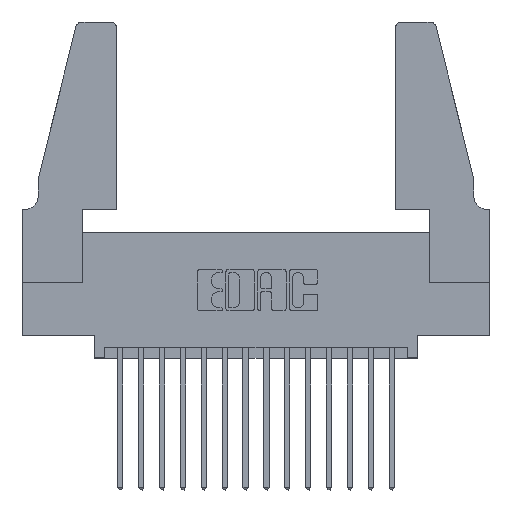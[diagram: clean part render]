
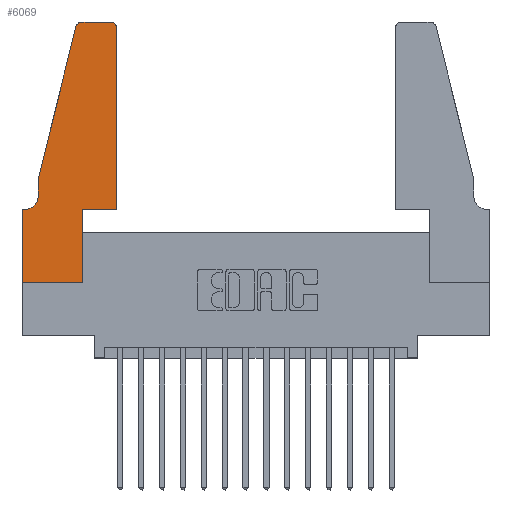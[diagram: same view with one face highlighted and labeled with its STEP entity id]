
A CAD part, top view. The second image highlights one B-rep face of the part: STEP entity #6069.
In plain terms, the highlighted planar face has unit normal (0, 0, 1).
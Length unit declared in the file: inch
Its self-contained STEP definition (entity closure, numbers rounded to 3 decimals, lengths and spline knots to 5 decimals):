
#523 = VERTEX_POINT ( 'NONE', #4623 ) ;
#659 = DIRECTION ( 'NONE',  ( -1., 0., 0. ) ) ;
#923 = DIRECTION ( 'NONE',  ( 1., 0., 0. ) ) ;
#1056 = EDGE_CURVE ( 'NONE', #14252, #4500, #13215, .T. ) ;
#1067 = VERTEX_POINT ( 'NONE', #11701 ) ;
#1222 = ORIENTED_EDGE ( 'NONE', *, *, #1919, .T. ) ;
#1332 = CARTESIAN_POINT ( 'NONE',  ( 0.0755, 0.5, 0.37 ) ) ;
#1691 = VERTEX_POINT ( 'NONE', #14984 ) ;
#1779 = CARTESIAN_POINT ( 'NONE',  ( 0., 0., 0.37 ) ) ;
#1919 = EDGE_CURVE ( 'NONE', #10856, #523, #10089, .T. ) ;
#2397 = VECTOR ( 'NONE', #659, 39.37008 ) ;
#2591 = CARTESIAN_POINT ( 'NONE',  ( 0.4505, 0.35, 0.37 ) ) ;
#2633 = FACE_OUTER_BOUND ( 'NONE', #6565, .T. ) ;
#2664 = ORIENTED_EDGE ( 'NONE', *, *, #2815, .T. ) ;
#2815 = EDGE_CURVE ( 'NONE', #8486, #12716, #12316, .T. ) ;
#3139 = VERTEX_POINT ( 'NONE', #11170 ) ;
#3157 = CARTESIAN_POINT ( 'NONE',  ( 0.284, 1.22, 0.37 ) ) ;
#3527 = VECTOR ( 'NONE', #16235, 39.37008 ) ;
#3567 = CARTESIAN_POINT ( 'NONE',  ( 0.2865, 0.35, 0.37 ) ) ;
#3930 = ORIENTED_EDGE ( 'NONE', *, *, #1056, .T. ) ;
#4178 = CARTESIAN_POINT ( 'NONE',  ( 0.4505, 0.35, 0.37 ) ) ;
#4500 = VERTEX_POINT ( 'NONE', #4964 ) ;
#4520 = DIRECTION ( 'NONE',  ( 1., 0., 0. ) ) ;
#4623 = CARTESIAN_POINT ( 'NONE',  ( 0.2865, 0.35, 0.37 ) ) ;
#4757 = EDGE_CURVE ( 'NONE', #12716, #1067, #7032, .T. ) ;
#4780 = ORIENTED_EDGE ( 'NONE', *, *, #6466, .T. ) ;
#4964 = CARTESIAN_POINT ( 'NONE',  ( 0., 0.35, 0.37 ) ) ;
#5061 = EDGE_CURVE ( 'NONE', #3139, #9304, #5195, .T. ) ;
#5195 = LINE ( 'NONE', #2591, #15659 ) ;
#5306 = EDGE_CURVE ( 'NONE', #13764, #8486, #14652, .T. ) ;
#5380 = CIRCLE ( 'NONE', #12347, 0.07 ) ;
#5598 = DIRECTION ( 'NONE',  ( 0., 0., -1. ) ) ;
#5767 = VECTOR ( 'NONE', #11004, 39.37008 ) ;
#5789 = ORIENTED_EDGE ( 'NONE', *, *, #15074, .T. ) ;
#5987 = DIRECTION ( 'NONE',  ( 0., 0., 1. ) ) ;
#6069 = ADVANCED_FACE ( 'NONE', ( #2633 ), #13903, .T. ) ;
#6105 = DIRECTION ( 'NONE',  ( 0., 0., 1. ) ) ;
#6466 = EDGE_CURVE ( 'NONE', #523, #3139, #11343, .T. ) ;
#6565 = EDGE_LOOP ( 'NONE', ( #5789, #9297, #2664, #6605, #17077, #3930, #7438, #14859, #1222, #4780, #9094, #16058 ) ) ;
#6605 = ORIENTED_EDGE ( 'NONE', *, *, #4757, .T. ) ;
#7032 = LINE ( 'NONE', #14943, #3527 ) ;
#7135 = CARTESIAN_POINT ( 'NONE',  ( 0.284, 1.25, 0.37 ) ) ;
#7438 = ORIENTED_EDGE ( 'NONE', *, *, #14861, .T. ) ;
#7891 = CARTESIAN_POINT ( 'NONE',  ( 0.2865, 0., 0.37 ) ) ;
#8262 = AXIS2_PLACEMENT_3D ( 'NONE', #3157, #12433, #4520 ) ;
#8486 = VERTEX_POINT ( 'NONE', #14629 ) ;
#8613 = CARTESIAN_POINT ( 'NONE',  ( 0.4505, 1.22, 0.37 ) ) ;
#8853 = CARTESIAN_POINT ( 'NONE',  ( 0., 0., 0.37 ) ) ;
#9094 = ORIENTED_EDGE ( 'NONE', *, *, #5061, .T. ) ;
#9297 = ORIENTED_EDGE ( 'NONE', *, *, #5306, .T. ) ;
#9304 = VERTEX_POINT ( 'NONE', #8613 ) ;
#10089 = LINE ( 'NONE', #3567, #10508 ) ;
#10294 = LINE ( 'NONE', #16446, #2397 ) ;
#10508 = VECTOR ( 'NONE', #11502, 39.37008 ) ;
#10517 = VECTOR ( 'NONE', #14729, 39.37008 ) ;
#10621 = EDGE_CURVE ( 'NONE', #9304, #1691, #16713, .T. ) ;
#10639 = CARTESIAN_POINT ( 'NONE',  ( 0.0755, 0.35, 0.37 ) ) ;
#10856 = VERTEX_POINT ( 'NONE', #7891 ) ;
#11004 = DIRECTION ( 'NONE',  ( -1., 0., 0. ) ) ;
#11170 = CARTESIAN_POINT ( 'NONE',  ( 0.4505, 0.35, 0.37 ) ) ;
#11256 = CARTESIAN_POINT ( 'NONE',  ( 0., 0.35, 0.37 ) ) ;
#11343 = LINE ( 'NONE', #4178, #10517 ) ;
#11360 = EDGE_CURVE ( 'NONE', #12328, #10856, #12247, .T. ) ;
#11502 = DIRECTION ( 'NONE',  ( 0., 1., 0. ) ) ;
#11701 = CARTESIAN_POINT ( 'NONE',  ( 0.0755, 0.42, 0.37 ) ) ;
#11766 = AXIS2_PLACEMENT_3D ( 'NONE', #14033, #6105, #15302 ) ;
#11899 = VECTOR ( 'NONE', #14556, 39.37008 ) ;
#12085 = CARTESIAN_POINT ( 'NONE',  ( 0., 0., 0.37 ) ) ;
#12247 = LINE ( 'NONE', #8853, #12670 ) ;
#12316 = LINE ( 'NONE', #1332, #11899 ) ;
#12328 = VERTEX_POINT ( 'NONE', #1779 ) ;
#12347 = AXIS2_PLACEMENT_3D ( 'NONE', #13510, #5598, #14812 ) ;
#12433 = DIRECTION ( 'NONE',  ( 0., 0., 1. ) ) ;
#12670 = VECTOR ( 'NONE', #923, 39.37008 ) ;
#12716 = VERTEX_POINT ( 'NONE', #15640 ) ;
#13186 = LINE ( 'NONE', #12085, #16205 ) ;
#13215 = LINE ( 'NONE', #10639, #5767 ) ;
#13510 = CARTESIAN_POINT ( 'NONE',  ( 0.0055, 0.42, 0.37 ) ) ;
#13600 = EDGE_CURVE ( 'NONE', #1067, #14252, #5380, .T. ) ;
#13764 = VERTEX_POINT ( 'NONE', #7135 ) ;
#13903 = PLANE ( 'NONE',  #14671 ) ;
#14033 = CARTESIAN_POINT ( 'NONE',  ( 0.4205, 1.22, 0.37 ) ) ;
#14252 = VERTEX_POINT ( 'NONE', #16073 ) ;
#14556 = DIRECTION ( 'NONE',  ( -0.239, -0.971, 0. ) ) ;
#14629 = CARTESIAN_POINT ( 'NONE',  ( 0.25487, 1.22718, 0.37 ) ) ;
#14652 = CIRCLE ( 'NONE', #8262, 0.03 ) ;
#14658 = DIRECTION ( 'NONE',  ( 0., -1., 0. ) ) ;
#14671 = AXIS2_PLACEMENT_3D ( 'NONE', #11256, #5987, #15182 ) ;
#14729 = DIRECTION ( 'NONE',  ( 1., 0., 0. ) ) ;
#14812 = DIRECTION ( 'NONE',  ( -1., 0., 0. ) ) ;
#14859 = ORIENTED_EDGE ( 'NONE', *, *, #11360, .T. ) ;
#14861 = EDGE_CURVE ( 'NONE', #4500, #12328, #13186, .T. ) ;
#14943 = CARTESIAN_POINT ( 'NONE',  ( 0.0755, 0.5, 0.37 ) ) ;
#14984 = CARTESIAN_POINT ( 'NONE',  ( 0.4205, 1.25, 0.37 ) ) ;
#15074 = EDGE_CURVE ( 'NONE', #1691, #13764, #10294, .T. ) ;
#15182 = DIRECTION ( 'NONE',  ( 1., 0., 0. ) ) ;
#15302 = DIRECTION ( 'NONE',  ( 1., 0., 0. ) ) ;
#15640 = CARTESIAN_POINT ( 'NONE',  ( 0.0755, 0.5, 0.37 ) ) ;
#15659 = VECTOR ( 'NONE', #15716, 39.37008 ) ;
#15716 = DIRECTION ( 'NONE',  ( 0., 1., 0. ) ) ;
#16058 = ORIENTED_EDGE ( 'NONE', *, *, #10621, .T. ) ;
#16073 = CARTESIAN_POINT ( 'NONE',  ( 0.0055, 0.35, 0.37 ) ) ;
#16205 = VECTOR ( 'NONE', #14658, 39.37008 ) ;
#16235 = DIRECTION ( 'NONE',  ( 0., -1., 0. ) ) ;
#16446 = CARTESIAN_POINT ( 'NONE',  ( 0.2605, 1.25, 0.37 ) ) ;
#16713 = CIRCLE ( 'NONE', #11766, 0.03 ) ;
#17077 = ORIENTED_EDGE ( 'NONE', *, *, #13600, .T. ) ;
